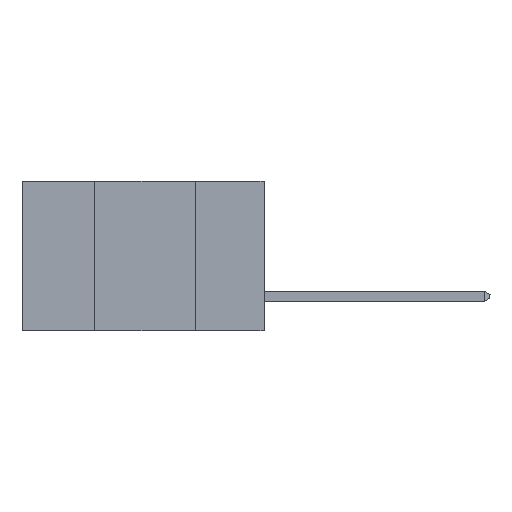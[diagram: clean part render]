
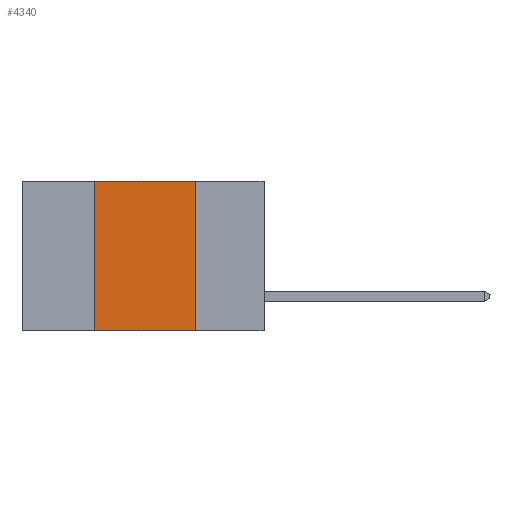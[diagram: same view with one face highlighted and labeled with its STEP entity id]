
A CAD part, left-side view. The second image highlights one B-rep face of the part: STEP entity #4340.
In plain terms, the highlighted planar face has unit normal (-1, 0, 0).
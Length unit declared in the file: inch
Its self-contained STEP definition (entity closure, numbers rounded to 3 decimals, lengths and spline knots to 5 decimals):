
#44 = VECTOR ( 'NONE', #10187, 39.37008 ) ;
#175 = EDGE_CURVE ( 'NONE', #4273, #2756, #13539, .T. ) ;
#316 = EDGE_CURVE ( 'NONE', #4273, #8299, #803, .T. ) ;
#784 = CARTESIAN_POINT ( 'NONE',  ( 0., 0.17, -0.37 ) ) ;
#803 = LINE ( 'NONE', #4429, #44 ) ;
#1128 = DIRECTION ( 'NONE',  ( 0., 0., -1. ) ) ;
#1315 = VECTOR ( 'NONE', #1128, 39.37008 ) ;
#1587 = CARTESIAN_POINT ( 'NONE',  ( 0., 0.42, 0. ) ) ;
#2071 = DIRECTION ( 'NONE',  ( 0., -1., 0. ) ) ;
#2260 = ORIENTED_EDGE ( 'NONE', *, *, #14455, .F. ) ;
#2283 = CARTESIAN_POINT ( 'NONE',  ( 0., 0.17, -0.37 ) ) ;
#2756 = VERTEX_POINT ( 'NONE', #784 ) ;
#3149 = ORIENTED_EDGE ( 'NONE', *, *, #15108, .F. ) ;
#3463 = CARTESIAN_POINT ( 'NONE',  ( 0., 0.17, 0. ) ) ;
#3979 = CARTESIAN_POINT ( 'NONE',  ( 0., 0.6, -0.37 ) ) ;
#4273 = VERTEX_POINT ( 'NONE', #5776 ) ;
#4340 = ADVANCED_FACE ( 'NONE', ( #11708 ), #15106, .F. ) ;
#4429 = CARTESIAN_POINT ( 'NONE',  ( 0., 0.42, -0.37 ) ) ;
#5648 = ORIENTED_EDGE ( 'NONE', *, *, #175, .T. ) ;
#5776 = CARTESIAN_POINT ( 'NONE',  ( 0., 0.42, -0.37 ) ) ;
#6933 = CARTESIAN_POINT ( 'NONE',  ( 0., 0.6, 0. ) ) ;
#8299 = VERTEX_POINT ( 'NONE', #1587 ) ;
#8327 = EDGE_LOOP ( 'NONE', ( #2260, #3149, #12615, #5648 ) ) ;
#9174 = CARTESIAN_POINT ( 'NONE',  ( 0., 0.6, 0. ) ) ;
#9306 = LINE ( 'NONE', #2283, #1315 ) ;
#10187 = DIRECTION ( 'NONE',  ( 0., 0., 1. ) ) ;
#10549 = DIRECTION ( 'NONE',  ( 0., 0., -1. ) ) ;
#11708 = FACE_OUTER_BOUND ( 'NONE', #8327, .T. ) ;
#12168 = VECTOR ( 'NONE', #2071, 39.37008 ) ;
#12615 = ORIENTED_EDGE ( 'NONE', *, *, #316, .F. ) ;
#12633 = LINE ( 'NONE', #6933, #12168 ) ;
#13451 = DIRECTION ( 'NONE',  ( 0., -1., 0. ) ) ;
#13539 = LINE ( 'NONE', #3979, #14664 ) ;
#13881 = DIRECTION ( 'NONE',  ( 1., 0., 0. ) ) ;
#14196 = AXIS2_PLACEMENT_3D ( 'NONE', #9174, #13881, #10549 ) ;
#14455 = EDGE_CURVE ( 'NONE', #15016, #2756, #9306, .T. ) ;
#14664 = VECTOR ( 'NONE', #13451, 39.37008 ) ;
#15016 = VERTEX_POINT ( 'NONE', #3463 ) ;
#15106 = PLANE ( 'NONE',  #14196 ) ;
#15108 = EDGE_CURVE ( 'NONE', #8299, #15016, #12633, .T. ) ;
